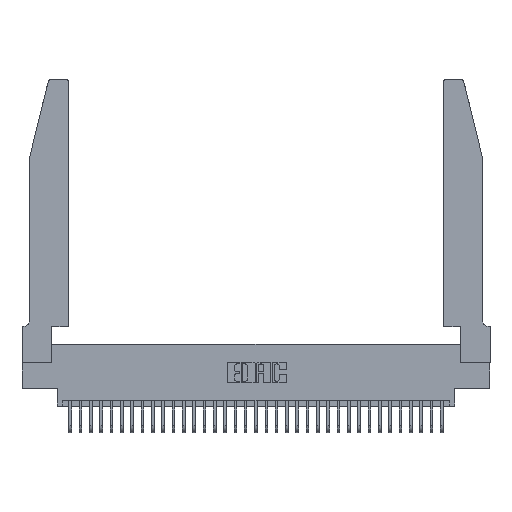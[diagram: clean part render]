
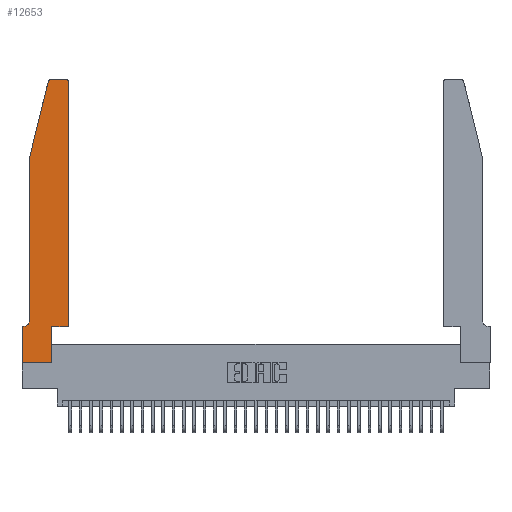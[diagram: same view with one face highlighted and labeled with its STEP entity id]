
A CAD part, top view. The second image highlights one B-rep face of the part: STEP entity #12653.
In plain terms, the highlighted planar face has unit normal (0, 0, 1).
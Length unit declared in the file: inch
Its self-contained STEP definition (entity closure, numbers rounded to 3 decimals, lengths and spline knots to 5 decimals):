
#290 = VECTOR ( 'NONE', #33217, 39.37008 ) ;
#964 = CIRCLE ( 'NONE', #36134, 0.03 ) ;
#1137 = EDGE_CURVE ( 'NONE', #30659, #16361, #27528, .T. ) ;
#1512 = PLANE ( 'NONE',  #28825 ) ;
#1713 = CARTESIAN_POINT ( 'NONE',  ( 0., 0., 0.37 ) ) ;
#2552 = CARTESIAN_POINT ( 'NONE',  ( 0.4505, 0.35, 0.37 ) ) ;
#3359 = DIRECTION ( 'NONE',  ( -0.239, -0.971, 0. ) ) ;
#3390 = VERTEX_POINT ( 'NONE', #26089 ) ;
#3720 = ORIENTED_EDGE ( 'NONE', *, *, #34166, .T. ) ;
#4033 = LINE ( 'NONE', #27793, #32164 ) ;
#4218 = VECTOR ( 'NONE', #13052, 39.37008 ) ;
#4326 = DIRECTION ( 'NONE',  ( 1., 0., 0. ) ) ;
#4385 = AXIS2_PLACEMENT_3D ( 'NONE', #10628, #30304, #13464 ) ;
#6063 = CARTESIAN_POINT ( 'NONE',  ( 0.0755, 2., 0.37 ) ) ;
#6101 = ORIENTED_EDGE ( 'NONE', *, *, #26591, .T. ) ;
#6271 = VECTOR ( 'NONE', #16750, 39.37008 ) ;
#6924 = CARTESIAN_POINT ( 'NONE',  ( 0.0755, 0.42, 0.37 ) ) ;
#7888 = CARTESIAN_POINT ( 'NONE',  ( 0.284, 2.75, 0.37 ) ) ;
#8606 = CARTESIAN_POINT ( 'NONE',  ( 0.4205, 2.72, 0.37 ) ) ;
#8762 = VERTEX_POINT ( 'NONE', #7888 ) ;
#9067 = VERTEX_POINT ( 'NONE', #34400 ) ;
#10104 = CARTESIAN_POINT ( 'NONE',  ( 0.4505, 2.72, 0.37 ) ) ;
#10149 = EDGE_CURVE ( 'NONE', #9067, #33272, #34329, .T. ) ;
#10355 = ORIENTED_EDGE ( 'NONE', *, *, #32641, .T. ) ;
#10628 = CARTESIAN_POINT ( 'NONE',  ( 0.0055, 0.42, 0.37 ) ) ;
#10788 = VERTEX_POINT ( 'NONE', #18613 ) ;
#11445 = DIRECTION ( 'NONE',  ( 1., 0., 0. ) ) ;
#11782 = DIRECTION ( 'NONE',  ( 0., 1., 0. ) ) ;
#11793 = ORIENTED_EDGE ( 'NONE', *, *, #10149, .T. ) ;
#11980 = VECTOR ( 'NONE', #3359, 39.37008 ) ;
#12303 = EDGE_CURVE ( 'NONE', #36103, #8762, #18474, .T. ) ;
#12653 = ADVANCED_FACE ( 'NONE', ( #21965 ), #1512, .T. ) ;
#13052 = DIRECTION ( 'NONE',  ( 0., -1., 0. ) ) ;
#13115 = ORIENTED_EDGE ( 'NONE', *, *, #33019, .T. ) ;
#13135 = DIRECTION ( 'NONE',  ( 0., 0., 1. ) ) ;
#13356 = EDGE_CURVE ( 'NONE', #21151, #32943, #28842, .T. ) ;
#13464 = DIRECTION ( 'NONE',  ( -1., 0., 0. ) ) ;
#13760 = LINE ( 'NONE', #22292, #6271 ) ;
#13887 = VECTOR ( 'NONE', #26914, 39.37008 ) ;
#14036 = ORIENTED_EDGE ( 'NONE', *, *, #35301, .T. ) ;
#14045 = DIRECTION ( 'NONE',  ( -1., 0., 0. ) ) ;
#14389 = CARTESIAN_POINT ( 'NONE',  ( 0.2865, 0., 0.37 ) ) ;
#14936 = EDGE_LOOP ( 'NONE', ( #26003, #32559, #3720, #10355, #16581, #27576, #17039, #31514, #13115, #11793, #6101, #14036 ) ) ;
#15932 = CIRCLE ( 'NONE', #33414, 0.03 ) ;
#15951 = EDGE_CURVE ( 'NONE', #16361, #21151, #13760, .T. ) ;
#16361 = VERTEX_POINT ( 'NONE', #18820 ) ;
#16581 = ORIENTED_EDGE ( 'NONE', *, *, #34601, .T. ) ;
#16702 = VECTOR ( 'NONE', #14045, 39.37008 ) ;
#16750 = DIRECTION ( 'NONE',  ( 0., -1., 0. ) ) ;
#17039 = ORIENTED_EDGE ( 'NONE', *, *, #15951, .T. ) ;
#18474 = LINE ( 'NONE', #22450, #16702 ) ;
#18569 = VECTOR ( 'NONE', #25030, 39.37008 ) ;
#18574 = CARTESIAN_POINT ( 'NONE',  ( 0., 0., 0.37 ) ) ;
#18613 = CARTESIAN_POINT ( 'NONE',  ( 0.25487, 2.72718, 0.37 ) ) ;
#18820 = CARTESIAN_POINT ( 'NONE',  ( 0., 0.35, 0.37 ) ) ;
#19000 = VERTEX_POINT ( 'NONE', #6924 ) ;
#19536 = LINE ( 'NONE', #6063, #11980 ) ;
#19841 = VERTEX_POINT ( 'NONE', #10104 ) ;
#21151 = VERTEX_POINT ( 'NONE', #18574 ) ;
#21194 = DIRECTION ( 'NONE',  ( 0., 0., 1. ) ) ;
#21811 = LINE ( 'NONE', #28774, #29270 ) ;
#21965 = FACE_OUTER_BOUND ( 'NONE', #14936, .T. ) ;
#22292 = CARTESIAN_POINT ( 'NONE',  ( 0., 0., 0.37 ) ) ;
#22450 = CARTESIAN_POINT ( 'NONE',  ( 0.2605, 2.75, 0.37 ) ) ;
#23217 = CARTESIAN_POINT ( 'NONE',  ( 0.4205, 2.75, 0.37 ) ) ;
#24270 = CARTESIAN_POINT ( 'NONE',  ( 0.0755, 2., 0.37 ) ) ;
#25030 = DIRECTION ( 'NONE',  ( 1., 0., 0. ) ) ;
#25062 = DIRECTION ( 'NONE',  ( 0., 1., 0. ) ) ;
#26003 = ORIENTED_EDGE ( 'NONE', *, *, #12303, .T. ) ;
#26089 = CARTESIAN_POINT ( 'NONE',  ( 0.0755, 2., 0.37 ) ) ;
#26404 = EDGE_CURVE ( 'NONE', #8762, #10788, #15932, .T. ) ;
#26591 = EDGE_CURVE ( 'NONE', #33272, #19841, #4033, .T. ) ;
#26914 = DIRECTION ( 'NONE',  ( 1., 0., 0. ) ) ;
#27528 = LINE ( 'NONE', #33095, #290 ) ;
#27576 = ORIENTED_EDGE ( 'NONE', *, *, #1137, .T. ) ;
#27793 = CARTESIAN_POINT ( 'NONE',  ( 0.4505, 0.35, 0.37 ) ) ;
#28328 = DIRECTION ( 'NONE',  ( 0., 0., 1. ) ) ;
#28699 = CIRCLE ( 'NONE', #4385, 0.07 ) ;
#28774 = CARTESIAN_POINT ( 'NONE',  ( 0.2865, 0.35, 0.37 ) ) ;
#28825 = AXIS2_PLACEMENT_3D ( 'NONE', #32341, #21194, #4326 ) ;
#28842 = LINE ( 'NONE', #1713, #13887 ) ;
#29270 = VECTOR ( 'NONE', #11782, 39.37008 ) ;
#29989 = CARTESIAN_POINT ( 'NONE',  ( 0.284, 2.72, 0.37 ) ) ;
#30304 = DIRECTION ( 'NONE',  ( 0., 0., -1. ) ) ;
#30659 = VERTEX_POINT ( 'NONE', #34706 ) ;
#31514 = ORIENTED_EDGE ( 'NONE', *, *, #13356, .T. ) ;
#32164 = VECTOR ( 'NONE', #25062, 39.37008 ) ;
#32341 = CARTESIAN_POINT ( 'NONE',  ( 0., 0.35, 0.37 ) ) ;
#32559 = ORIENTED_EDGE ( 'NONE', *, *, #26404, .T. ) ;
#32641 = EDGE_CURVE ( 'NONE', #3390, #19000, #34087, .T. ) ;
#32800 = DIRECTION ( 'NONE',  ( 1., 0., 0. ) ) ;
#32943 = VERTEX_POINT ( 'NONE', #14389 ) ;
#33019 = EDGE_CURVE ( 'NONE', #32943, #9067, #21811, .T. ) ;
#33095 = CARTESIAN_POINT ( 'NONE',  ( 0.0755, 0.35, 0.37 ) ) ;
#33217 = DIRECTION ( 'NONE',  ( -1., 0., 0. ) ) ;
#33272 = VERTEX_POINT ( 'NONE', #35569 ) ;
#33414 = AXIS2_PLACEMENT_3D ( 'NONE', #29989, #13135, #32800 ) ;
#34087 = LINE ( 'NONE', #24270, #4218 ) ;
#34166 = EDGE_CURVE ( 'NONE', #10788, #3390, #19536, .T. ) ;
#34329 = LINE ( 'NONE', #2552, #18569 ) ;
#34400 = CARTESIAN_POINT ( 'NONE',  ( 0.2865, 0.35, 0.37 ) ) ;
#34601 = EDGE_CURVE ( 'NONE', #19000, #30659, #28699, .T. ) ;
#34706 = CARTESIAN_POINT ( 'NONE',  ( 0.0055, 0.35, 0.37 ) ) ;
#35301 = EDGE_CURVE ( 'NONE', #19841, #36103, #964, .T. ) ;
#35569 = CARTESIAN_POINT ( 'NONE',  ( 0.4505, 0.35, 0.37 ) ) ;
#36103 = VERTEX_POINT ( 'NONE', #23217 ) ;
#36134 = AXIS2_PLACEMENT_3D ( 'NONE', #8606, #28328, #11445 ) ;
